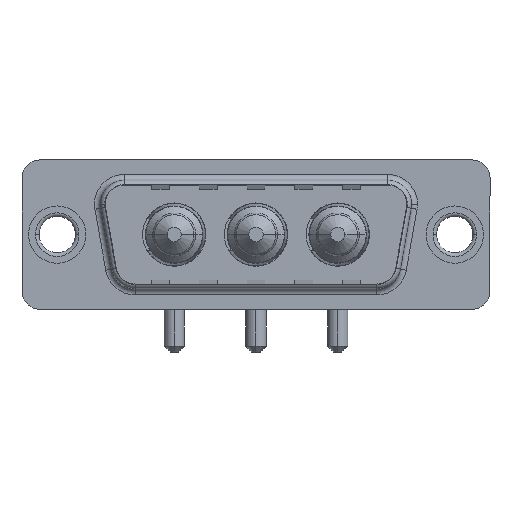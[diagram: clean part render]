
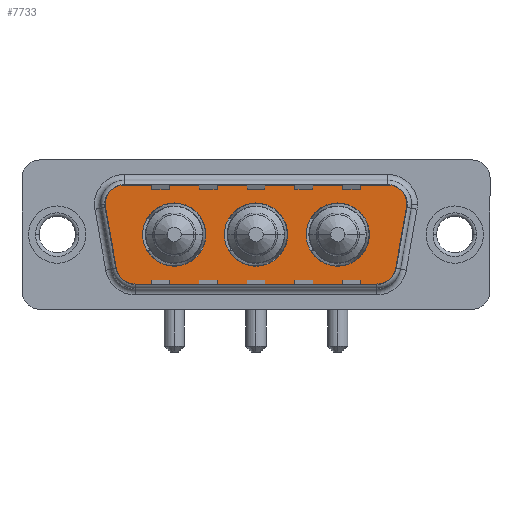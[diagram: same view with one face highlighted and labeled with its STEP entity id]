
A CAD part, top view. The second image highlights one B-rep face of the part: STEP entity #7733.
In plain terms, the highlighted planar face has unit normal (0, 0, 1).
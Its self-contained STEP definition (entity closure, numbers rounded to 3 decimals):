
#4 = CIRCLE ( 'NONE', #7534, 2.65 ) ;
#144 = VERTEX_POINT ( 'NONE', #2296 ) ;
#234 = DIRECTION ( 'NONE',  ( 0.174, -0.985, 0. ) ) ;
#297 = DIRECTION ( 'NONE',  ( -1., 0., 0. ) ) ;
#352 = ORIENTED_EDGE ( 'NONE', *, *, #1584, .T. ) ;
#363 = VECTOR ( 'NONE', #234, 1000. ) ;
#365 = CARTESIAN_POINT ( 'NONE',  ( 6.434, -2.9, 0. ) ) ;
#371 = DIRECTION ( 'NONE',  ( 1., 0., 0. ) ) ;
#373 = CARTESIAN_POINT ( 'NONE',  ( 27.889, 4.9, 0. ) ) ;
#391 = DIRECTION ( 'NONE',  ( -1., 0., 0. ) ) ;
#399 = VERTEX_POINT ( 'NONE', #7015 ) ;
#501 = CIRCLE ( 'NONE', #685, 2.65 ) ;
#529 = EDGE_CURVE ( 'NONE', #8031, #6920, #7450, .T. ) ;
#593 = VERTEX_POINT ( 'NONE', #4978 ) ;
#607 = ORIENTED_EDGE ( 'NONE', *, *, #10893, .T. ) ;
#685 = AXIS2_PLACEMENT_3D ( 'NONE', #10049, #3248, #5674 ) ;
#761 = CIRCLE ( 'NONE', #8474, 2.65 ) ;
#974 = ORIENTED_EDGE ( 'NONE', *, *, #8349, .T. ) ;
#975 = EDGE_CURVE ( 'NONE', #593, #4126, #4, .T. ) ;
#981 = CARTESIAN_POINT ( 'NONE',  ( 27.889, 2.9, 0. ) ) ;
#1260 = CARTESIAN_POINT ( 'NONE',  ( 16.65, 0., 0. ) ) ;
#1306 = CARTESIAN_POINT ( 'NONE',  ( 23.5, 0., 0. ) ) ;
#1368 = DIRECTION ( 'NONE',  ( 1., 0., 0. ) ) ;
#1460 = EDGE_CURVE ( 'NONE', #6714, #10216, #9558, .T. ) ;
#1570 = DIRECTION ( 'NONE',  ( 0.174, 0.985, 0. ) ) ;
#1584 = EDGE_CURVE ( 'NONE', #6920, #2924, #2409, .T. ) ;
#2064 = AXIS2_PLACEMENT_3D ( 'NONE', #3902, #5811, #2162 ) ;
#2162 = DIRECTION ( 'NONE',  ( 1., 0., 0. ) ) ;
#2296 = CARTESIAN_POINT ( 'NONE',  ( 5.411, 4.9, 0. ) ) ;
#2331 = CARTESIAN_POINT ( 'NONE',  ( 6.434, -4.9, 0. ) ) ;
#2409 = LINE ( 'NONE', #8590, #6639 ) ;
#2824 = CIRCLE ( 'NONE', #7847, 2.65 ) ;
#2832 = ORIENTED_EDGE ( 'NONE', *, *, #4469, .T. ) ;
#2924 = VERTEX_POINT ( 'NONE', #6009 ) ;
#3025 = DIRECTION ( 'NONE',  ( 0., 0., 1. ) ) ;
#3248 = DIRECTION ( 'NONE',  ( 0., 0., 1. ) ) ;
#3251 = CARTESIAN_POINT ( 'NONE',  ( 28.836, -3.247, 0. ) ) ;
#3303 = EDGE_CURVE ( 'NONE', #4660, #9793, #9718, .T. ) ;
#3523 = ORIENTED_EDGE ( 'NONE', *, *, #7595, .F. ) ;
#3618 = DIRECTION ( 'NONE',  ( 0., 0., 1. ) ) ;
#3686 = DIRECTION ( 'NONE',  ( 0., 0., 1. ) ) ;
#3713 = CARTESIAN_POINT ( 'NONE',  ( 6.434, -4.9, 0. ) ) ;
#3750 = DIRECTION ( 'NONE',  ( 0., 0., 1. ) ) ;
#3773 = EDGE_LOOP ( 'NONE', ( #7321, #352, #2832, #974, #607, #5241, #5753, #8264, #5059 ) ) ;
#3902 = CARTESIAN_POINT ( 'NONE',  ( 26.866, -2.9, 0. ) ) ;
#4017 = CARTESIAN_POINT ( 'NONE',  ( 5.411, 2.9, 0. ) ) ;
#4126 = VERTEX_POINT ( 'NONE', #10008 ) ;
#4191 = DIRECTION ( 'NONE',  ( 1., 0., 0. ) ) ;
#4469 = EDGE_CURVE ( 'NONE', #2924, #4729, #8853, .T. ) ;
#4561 = CARTESIAN_POINT ( 'NONE',  ( 3.441, 2.553, 0. ) ) ;
#4609 = CARTESIAN_POINT ( 'NONE',  ( 27.889, 2.9, 0. ) ) ;
#4660 = VERTEX_POINT ( 'NONE', #9149 ) ;
#4729 = VERTEX_POINT ( 'NONE', #8633 ) ;
#4755 = CARTESIAN_POINT ( 'NONE',  ( 9.8, 0., 0. ) ) ;
#4805 = DIRECTION ( 'NONE',  ( 0., 0., 1. ) ) ;
#4861 = DIRECTION ( 'NONE',  ( 1., 0., 0. ) ) ;
#4944 = ORIENTED_EDGE ( 'NONE', *, *, #10682, .F. ) ;
#4978 = CARTESIAN_POINT ( 'NONE',  ( 14., 0., 0. ) ) ;
#4997 = VERTEX_POINT ( 'NONE', #373 ) ;
#5059 = ORIENTED_EDGE ( 'NONE', *, *, #10730, .T. ) ;
#5241 = ORIENTED_EDGE ( 'NONE', *, *, #7753, .T. ) ;
#5338 = EDGE_CURVE ( 'NONE', #399, #5434, #761, .T. ) ;
#5434 = VERTEX_POINT ( 'NONE', #10898 ) ;
#5492 = CIRCLE ( 'NONE', #6214, 2. ) ;
#5516 = VECTOR ( 'NONE', #8516, 1000. ) ;
#5522 = DIRECTION ( 'NONE',  ( 0., 0., 1. ) ) ;
#5541 = CARTESIAN_POINT ( 'NONE',  ( 9.8, 0., 0. ) ) ;
#5544 = DIRECTION ( 'NONE',  ( 1., 0., 0. ) ) ;
#5674 = DIRECTION ( 'NONE',  ( 1., 0., 0. ) ) ;
#5753 = ORIENTED_EDGE ( 'NONE', *, *, #1460, .T. ) ;
#5811 = DIRECTION ( 'NONE',  ( 0., 0., 1. ) ) ;
#5842 = CIRCLE ( 'NONE', #11036, 2. ) ;
#5878 = DIRECTION ( 'NONE',  ( 0., 0., 1. ) ) ;
#6009 = CARTESIAN_POINT ( 'NONE',  ( 29.859, 2.553, 0. ) ) ;
#6142 = EDGE_LOOP ( 'NONE', ( #4944, #10191 ) ) ;
#6214 = AXIS2_PLACEMENT_3D ( 'NONE', #981, #3750, #391 ) ;
#6286 = CARTESIAN_POINT ( 'NONE',  ( 3.441, 2.553, 0. ) ) ;
#6393 = ORIENTED_EDGE ( 'NONE', *, *, #5338, .F. ) ;
#6434 = FACE_BOUND ( 'NONE', #6142, .T. ) ;
#6443 = EDGE_LOOP ( 'NONE', ( #3523, #6393 ) ) ;
#6497 = CARTESIAN_POINT ( 'NONE',  ( 26.866, -2.9, 0. ) ) ;
#6560 = AXIS2_PLACEMENT_3D ( 'NONE', #9597, #3686, #10630 ) ;
#6639 = VECTOR ( 'NONE', #1570, 1000. ) ;
#6714 = VERTEX_POINT ( 'NONE', #4561 ) ;
#6920 = VERTEX_POINT ( 'NONE', #3251 ) ;
#7015 = CARTESIAN_POINT ( 'NONE',  ( 20.85, 0., 0. ) ) ;
#7059 = AXIS2_PLACEMENT_3D ( 'NONE', #4609, #3025, #297 ) ;
#7127 = VECTOR ( 'NONE', #4861, 1000. ) ;
#7317 = CARTESIAN_POINT ( 'NONE',  ( 12.45, 0., 0. ) ) ;
#7321 = ORIENTED_EDGE ( 'NONE', *, *, #529, .T. ) ;
#7446 = FACE_BOUND ( 'NONE', #7638, .T. ) ;
#7450 = CIRCLE ( 'NONE', #9428, 2. ) ;
#7534 = AXIS2_PLACEMENT_3D ( 'NONE', #1260, #8222, #371 ) ;
#7595 = EDGE_CURVE ( 'NONE', #5434, #399, #9781, .T. ) ;
#7638 = EDGE_LOOP ( 'NONE', ( #10545, #9295 ) ) ;
#7733 = ADVANCED_FACE ( 'NONE', ( #7446, #8228, #6434, #10074 ), #8342, .T. ) ;
#7753 = EDGE_CURVE ( 'NONE', #144, #6714, #11028, .T. ) ;
#7836 = DIRECTION ( 'NONE',  ( -1., 0., 0. ) ) ;
#7847 = AXIS2_PLACEMENT_3D ( 'NONE', #5541, #8965, #7960 ) ;
#7889 = CARTESIAN_POINT ( 'NONE',  ( 26.866, -4.9, 0. ) ) ;
#7932 = AXIS2_PLACEMENT_3D ( 'NONE', #4755, #5878, #4191 ) ;
#7960 = DIRECTION ( 'NONE',  ( 1., 0., 0. ) ) ;
#7963 = EDGE_CURVE ( 'NONE', #10216, #10185, #5842, .T. ) ;
#8031 = VERTEX_POINT ( 'NONE', #7889 ) ;
#8222 = DIRECTION ( 'NONE',  ( 0., 0., 1. ) ) ;
#8228 = FACE_BOUND ( 'NONE', #6443, .T. ) ;
#8264 = ORIENTED_EDGE ( 'NONE', *, *, #7963, .T. ) ;
#8342 = PLANE ( 'NONE',  #2064 ) ;
#8349 = EDGE_CURVE ( 'NONE', #4729, #4997, #5492, .T. ) ;
#8397 = DIRECTION ( 'NONE',  ( 1., 0., 0. ) ) ;
#8474 = AXIS2_PLACEMENT_3D ( 'NONE', #1306, #5522, #1368 ) ;
#8516 = DIRECTION ( 'NONE',  ( -1., 0., 0. ) ) ;
#8590 = CARTESIAN_POINT ( 'NONE',  ( 29.859, 2.553, 0. ) ) ;
#8633 = CARTESIAN_POINT ( 'NONE',  ( 29.889, 2.9, 0. ) ) ;
#8853 = CIRCLE ( 'NONE', #7059, 2. ) ;
#8965 = DIRECTION ( 'NONE',  ( 0., 0., 1. ) ) ;
#9149 = CARTESIAN_POINT ( 'NONE',  ( 7.15, 0., 0. ) ) ;
#9295 = ORIENTED_EDGE ( 'NONE', *, *, #975, .F. ) ;
#9428 = AXIS2_PLACEMENT_3D ( 'NONE', #6497, #9811, #5544 ) ;
#9558 = LINE ( 'NONE', #6286, #363 ) ;
#9597 = CARTESIAN_POINT ( 'NONE',  ( 23.5, 0., 0. ) ) ;
#9677 = EDGE_CURVE ( 'NONE', #4126, #593, #501, .T. ) ;
#9718 = CIRCLE ( 'NONE', #7932, 2.65 ) ;
#9781 = CIRCLE ( 'NONE', #6560, 2.65 ) ;
#9793 = VERTEX_POINT ( 'NONE', #7317 ) ;
#9811 = DIRECTION ( 'NONE',  ( 0., 0., 1. ) ) ;
#10008 = CARTESIAN_POINT ( 'NONE',  ( 19.3, 0., 0. ) ) ;
#10049 = CARTESIAN_POINT ( 'NONE',  ( 16.65, 0., 0. ) ) ;
#10074 = FACE_OUTER_BOUND ( 'NONE', #3773, .T. ) ;
#10076 = LINE ( 'NONE', #2331, #7127 ) ;
#10135 = CARTESIAN_POINT ( 'NONE',  ( 5.411, 4.9, 0. ) ) ;
#10137 = AXIS2_PLACEMENT_3D ( 'NONE', #4017, #4805, #8397 ) ;
#10185 = VERTEX_POINT ( 'NONE', #3713 ) ;
#10191 = ORIENTED_EDGE ( 'NONE', *, *, #3303, .F. ) ;
#10216 = VERTEX_POINT ( 'NONE', #10346 ) ;
#10346 = CARTESIAN_POINT ( 'NONE',  ( 4.464, -3.247, 0. ) ) ;
#10545 = ORIENTED_EDGE ( 'NONE', *, *, #9677, .F. ) ;
#10630 = DIRECTION ( 'NONE',  ( 1., 0., 0. ) ) ;
#10682 = EDGE_CURVE ( 'NONE', #9793, #4660, #2824, .T. ) ;
#10730 = EDGE_CURVE ( 'NONE', #10185, #8031, #10076, .T. ) ;
#10893 = EDGE_CURVE ( 'NONE', #4997, #144, #10914, .T. ) ;
#10898 = CARTESIAN_POINT ( 'NONE',  ( 26.15, 0., 0. ) ) ;
#10914 = LINE ( 'NONE', #10135, #5516 ) ;
#11028 = CIRCLE ( 'NONE', #10137, 2. ) ;
#11036 = AXIS2_PLACEMENT_3D ( 'NONE', #365, #3618, #7836 ) ;
